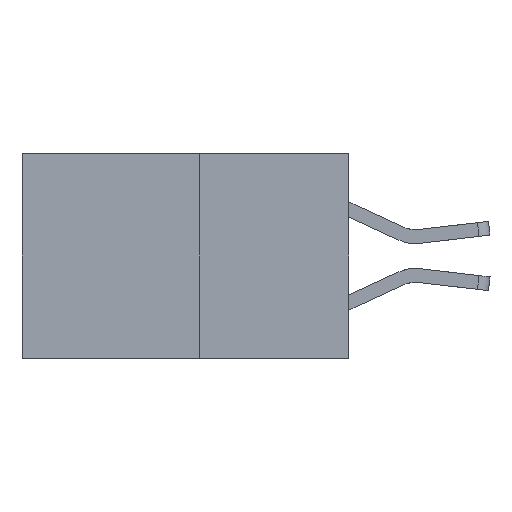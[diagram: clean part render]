
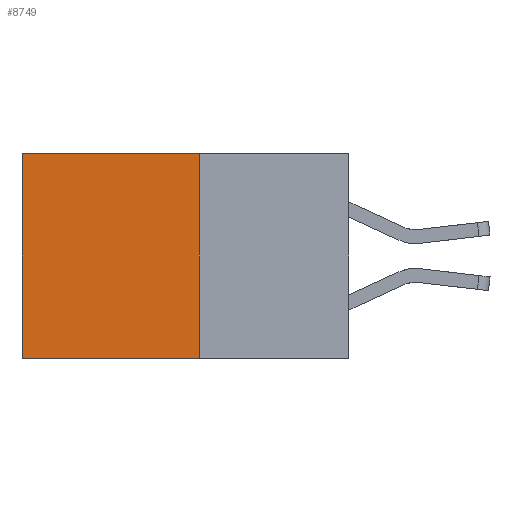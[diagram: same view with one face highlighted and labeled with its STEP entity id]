
A CAD part, left-side view. The second image highlights one B-rep face of the part: STEP entity #8749.
In plain terms, the highlighted planar face has unit normal (-1, 0, 0).
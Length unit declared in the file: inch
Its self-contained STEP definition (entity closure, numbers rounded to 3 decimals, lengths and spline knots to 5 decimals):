
#56 = DIRECTION ( 'NONE',  ( 0., 1., 0. ) ) ;
#166 = CARTESIAN_POINT ( 'NONE',  ( 0.277, 0.27, 0. ) ) ;
#348 = EDGE_CURVE ( 'NONE', #5322, #8554, #4193, .T. ) ;
#433 = LINE ( 'NONE', #10601, #7492 ) ;
#470 = CARTESIAN_POINT ( 'NONE',  ( 0.277, 0.27, 0. ) ) ;
#1342 = DIRECTION ( 'NONE',  ( 0., 0., -1. ) ) ;
#2366 = CARTESIAN_POINT ( 'NONE',  ( 0.277, 0.27, -0.37 ) ) ;
#2370 = CARTESIAN_POINT ( 'NONE',  ( 0.277, 0.59, -0.37 ) ) ;
#2429 = DIRECTION ( 'NONE',  ( 0., 0., -1. ) ) ;
#2458 = DIRECTION ( 'NONE',  ( 1., 0., 0. ) ) ;
#2489 = CARTESIAN_POINT ( 'NONE',  ( 0.277, 0.27, -0.37 ) ) ;
#2526 = PLANE ( 'NONE',  #8300 ) ;
#2614 = CARTESIAN_POINT ( 'NONE',  ( 0.277, 0.59, 0. ) ) ;
#4193 = LINE ( 'NONE', #2366, #11252 ) ;
#4310 = DIRECTION ( 'NONE',  ( 0., 0., -1. ) ) ;
#4325 = CARTESIAN_POINT ( 'NONE',  ( 0.277, 0.59, -0.37 ) ) ;
#4433 = VECTOR ( 'NONE', #4310, 39.37008 ) ;
#4731 = LINE ( 'NONE', #4325, #4433 ) ;
#4869 = CARTESIAN_POINT ( 'NONE',  ( 0.277, 0.27, -0.37 ) ) ;
#4945 = EDGE_CURVE ( 'NONE', #8554, #7677, #433, .T. ) ;
#5322 = VERTEX_POINT ( 'NONE', #470 ) ;
#6632 = EDGE_CURVE ( 'NONE', #5322, #8158, #7763, .T. ) ;
#7492 = VECTOR ( 'NONE', #11599, 39.37008 ) ;
#7677 = VERTEX_POINT ( 'NONE', #2370 ) ;
#7763 = LINE ( 'NONE', #166, #11740 ) ;
#8158 = VERTEX_POINT ( 'NONE', #2614 ) ;
#8300 = AXIS2_PLACEMENT_3D ( 'NONE', #2489, #2458, #2429 ) ;
#8554 = VERTEX_POINT ( 'NONE', #4869 ) ;
#8563 = EDGE_CURVE ( 'NONE', #8158, #7677, #4731, .T. ) ;
#8749 = ADVANCED_FACE ( 'NONE', ( #9675 ), #2526, .F. ) ;
#9675 = FACE_OUTER_BOUND ( 'NONE', #10400, .T. ) ;
#9849 = ORIENTED_EDGE ( 'NONE', *, *, #8563, .T. ) ;
#10400 = EDGE_LOOP ( 'NONE', ( #9849, #10432, #10643, #11380 ) ) ;
#10432 = ORIENTED_EDGE ( 'NONE', *, *, #4945, .F. ) ;
#10601 = CARTESIAN_POINT ( 'NONE',  ( 0.277, 0.27, -0.37 ) ) ;
#10643 = ORIENTED_EDGE ( 'NONE', *, *, #348, .F. ) ;
#11252 = VECTOR ( 'NONE', #1342, 39.37008 ) ;
#11380 = ORIENTED_EDGE ( 'NONE', *, *, #6632, .T. ) ;
#11599 = DIRECTION ( 'NONE',  ( 0., 1., 0. ) ) ;
#11740 = VECTOR ( 'NONE', #56, 39.37008 ) ;
